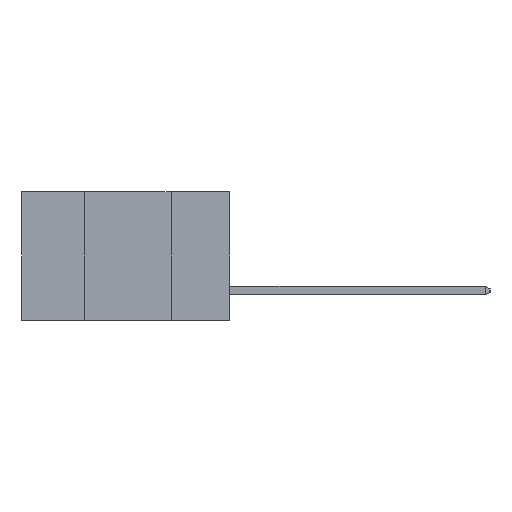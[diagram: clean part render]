
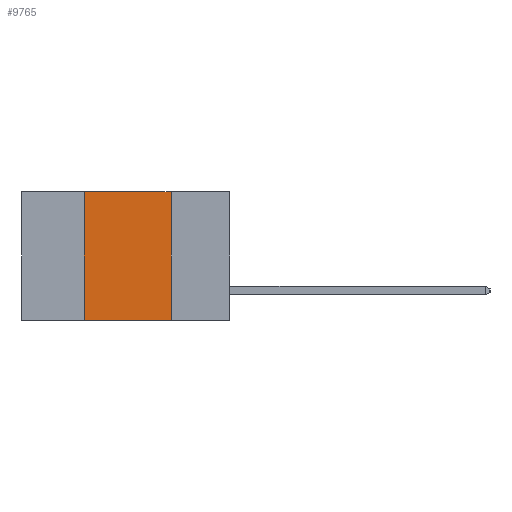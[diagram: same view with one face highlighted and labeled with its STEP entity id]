
A CAD part, left-side view. The second image highlights one B-rep face of the part: STEP entity #9765.
In plain terms, the highlighted planar face has unit normal (-1, 0, 0).
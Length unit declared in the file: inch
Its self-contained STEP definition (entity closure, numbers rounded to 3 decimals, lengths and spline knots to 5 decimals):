
#690 = CARTESIAN_POINT ( 'NONE',  ( 0., 0.17, 0. ) ) ;
#1716 = EDGE_CURVE ( 'NONE', #16971, #14967, #16795, .T. ) ;
#1800 = ORIENTED_EDGE ( 'NONE', *, *, #11807, .F. ) ;
#2252 = CARTESIAN_POINT ( 'NONE',  ( 0., 0.6, -0.37 ) ) ;
#3005 = AXIS2_PLACEMENT_3D ( 'NONE', #4920, #3534, #13390 ) ;
#3534 = DIRECTION ( 'NONE',  ( 1., 0., 0. ) ) ;
#4586 = ORIENTED_EDGE ( 'NONE', *, *, #14086, .F. ) ;
#4920 = CARTESIAN_POINT ( 'NONE',  ( 0., 0.6, 0. ) ) ;
#5590 = VECTOR ( 'NONE', #6611, 39.37008 ) ;
#6370 = VECTOR ( 'NONE', #13809, 39.37008 ) ;
#6611 = DIRECTION ( 'NONE',  ( 0., 0., -1. ) ) ;
#7090 = CARTESIAN_POINT ( 'NONE',  ( 0., 0.42, -0.37 ) ) ;
#7369 = FACE_OUTER_BOUND ( 'NONE', #13018, .T. ) ;
#7520 = CARTESIAN_POINT ( 'NONE',  ( 0., 0.17, 0. ) ) ;
#7688 = CARTESIAN_POINT ( 'NONE',  ( 0., 0.42, 0. ) ) ;
#8260 = VECTOR ( 'NONE', #16307, 39.37008 ) ;
#8414 = VERTEX_POINT ( 'NONE', #14640 ) ;
#9765 = ADVANCED_FACE ( 'NONE', ( #7369 ), #10673, .F. ) ;
#10454 = DIRECTION ( 'NONE',  ( 0., 0., 1. ) ) ;
#10673 = PLANE ( 'NONE',  #3005 ) ;
#10821 = ORIENTED_EDGE ( 'NONE', *, *, #1716, .F. ) ;
#11807 = EDGE_CURVE ( 'NONE', #14967, #17839, #17315, .T. ) ;
#12476 = CARTESIAN_POINT ( 'NONE',  ( 0., 0.6, 0. ) ) ;
#13018 = EDGE_LOOP ( 'NONE', ( #4586, #1800, #10821, #13775 ) ) ;
#13245 = VECTOR ( 'NONE', #10454, 39.37008 ) ;
#13390 = DIRECTION ( 'NONE',  ( 0., 0., -1. ) ) ;
#13505 = EDGE_CURVE ( 'NONE', #16971, #8414, #15596, .T. ) ;
#13775 = ORIENTED_EDGE ( 'NONE', *, *, #13505, .T. ) ;
#13809 = DIRECTION ( 'NONE',  ( 0., -1., 0. ) ) ;
#14086 = EDGE_CURVE ( 'NONE', #17839, #8414, #17000, .T. ) ;
#14640 = CARTESIAN_POINT ( 'NONE',  ( 0., 0.17, -0.37 ) ) ;
#14967 = VERTEX_POINT ( 'NONE', #15340 ) ;
#15340 = CARTESIAN_POINT ( 'NONE',  ( 0., 0.42, 0. ) ) ;
#15596 = LINE ( 'NONE', #2252, #8260 ) ;
#16307 = DIRECTION ( 'NONE',  ( 0., -1., 0. ) ) ;
#16795 = LINE ( 'NONE', #7688, #13245 ) ;
#16971 = VERTEX_POINT ( 'NONE', #7090 ) ;
#17000 = LINE ( 'NONE', #690, #5590 ) ;
#17315 = LINE ( 'NONE', #12476, #6370 ) ;
#17839 = VERTEX_POINT ( 'NONE', #7520 ) ;
